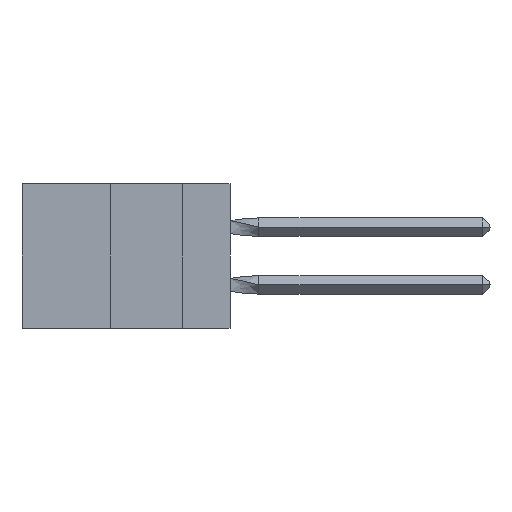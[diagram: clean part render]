
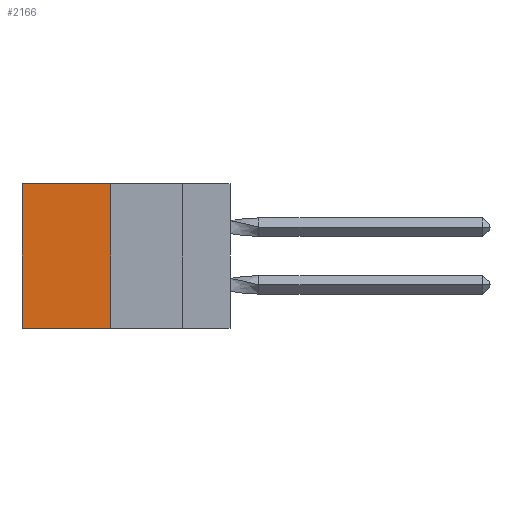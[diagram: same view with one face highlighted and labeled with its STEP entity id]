
A CAD part, left-side view. The second image highlights one B-rep face of the part: STEP entity #2166.
In plain terms, the highlighted planar face has unit normal (-1, 0, 0).
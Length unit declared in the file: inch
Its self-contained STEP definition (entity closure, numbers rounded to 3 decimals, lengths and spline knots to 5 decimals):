
#450 = CARTESIAN_POINT ( 'NONE',  ( 0.305, 0.413, -0.5 ) ) ;
#487 = VERTEX_POINT ( 'NONE', #16348 ) ;
#1035 = LINE ( 'NONE', #5480, #10567 ) ;
#1146 = PLANE ( 'NONE',  #13643 ) ;
#1666 = CARTESIAN_POINT ( 'NONE',  ( 0.305, 0.413, 0. ) ) ;
#2166 = ADVANCED_FACE ( 'NONE', ( #10816 ), #1146, .F. ) ;
#2347 = ORIENTED_EDGE ( 'NONE', *, *, #18069, .T. ) ;
#2351 = VERTEX_POINT ( 'NONE', #6070 ) ;
#2619 = CARTESIAN_POINT ( 'NONE',  ( 0.305, 0.413, -0.5 ) ) ;
#5397 = DIRECTION ( 'NONE',  ( 0., 0., -1. ) ) ;
#5480 = CARTESIAN_POINT ( 'NONE',  ( 0.305, 0.413, -0.5 ) ) ;
#6070 = CARTESIAN_POINT ( 'NONE',  ( 0.305, 0.72, 0. ) ) ;
#7620 = VECTOR ( 'NONE', #5397, 39.37008 ) ;
#8451 = VERTEX_POINT ( 'NONE', #450 ) ;
#9995 = DIRECTION ( 'NONE',  ( 0., 1., 0. ) ) ;
#10467 = VERTEX_POINT ( 'NONE', #1666 ) ;
#10567 = VECTOR ( 'NONE', #9995, 39.37008 ) ;
#10746 = ORIENTED_EDGE ( 'NONE', *, *, #15039, .T. ) ;
#10816 = FACE_OUTER_BOUND ( 'NONE', #15208, .T. ) ;
#11259 = DIRECTION ( 'NONE',  ( 1., 0., 0. ) ) ;
#11656 = VECTOR ( 'NONE', #15153, 39.37008 ) ;
#12574 = CARTESIAN_POINT ( 'NONE',  ( 0.305, 0.413, -0.5 ) ) ;
#12668 = LINE ( 'NONE', #18286, #17176 ) ;
#13485 = EDGE_CURVE ( 'NONE', #10467, #8451, #17336, .T. ) ;
#13643 = AXIS2_PLACEMENT_3D ( 'NONE', #2619, #11259, #17016 ) ;
#14761 = EDGE_CURVE ( 'NONE', #8451, #487, #1035, .T. ) ;
#14961 = CARTESIAN_POINT ( 'NONE',  ( 0.305, 0.72, -0.5 ) ) ;
#15039 = EDGE_CURVE ( 'NONE', #2351, #487, #15044, .T. ) ;
#15044 = LINE ( 'NONE', #14961, #11656 ) ;
#15153 = DIRECTION ( 'NONE',  ( 0., 0., -1. ) ) ;
#15208 = EDGE_LOOP ( 'NONE', ( #10746, #18128, #17117, #2347 ) ) ;
#16348 = CARTESIAN_POINT ( 'NONE',  ( 0.305, 0.72, -0.5 ) ) ;
#16933 = DIRECTION ( 'NONE',  ( 0., 1., 0. ) ) ;
#17016 = DIRECTION ( 'NONE',  ( 0., 0., -1. ) ) ;
#17117 = ORIENTED_EDGE ( 'NONE', *, *, #13485, .F. ) ;
#17176 = VECTOR ( 'NONE', #16933, 39.37008 ) ;
#17336 = LINE ( 'NONE', #12574, #7620 ) ;
#18069 = EDGE_CURVE ( 'NONE', #10467, #2351, #12668, .T. ) ;
#18128 = ORIENTED_EDGE ( 'NONE', *, *, #14761, .F. ) ;
#18286 = CARTESIAN_POINT ( 'NONE',  ( 0.305, 0.413, 0. ) ) ;
